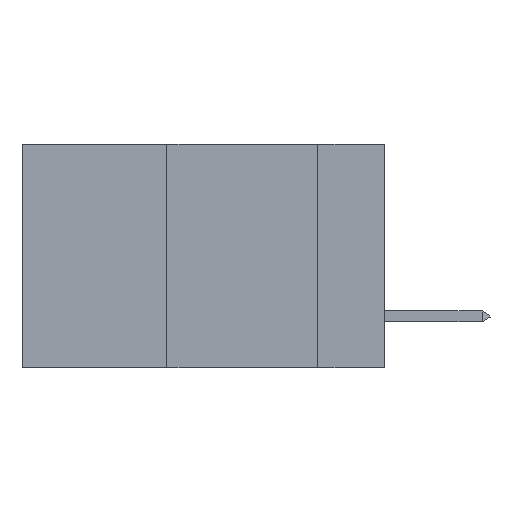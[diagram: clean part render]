
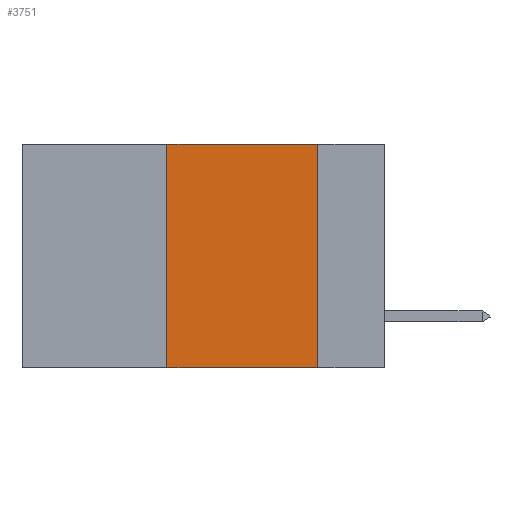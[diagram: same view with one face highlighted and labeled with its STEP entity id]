
A CAD part, left-side view. The second image highlights one B-rep face of the part: STEP entity #3751.
In plain terms, the highlighted planar face has unit normal (-1, 0, 0).
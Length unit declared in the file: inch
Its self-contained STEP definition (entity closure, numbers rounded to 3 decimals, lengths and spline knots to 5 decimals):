
#116 = DIRECTION ( 'NONE',  ( 0., 0., 1. ) ) ;
#193 = CARTESIAN_POINT ( 'NONE',  ( 0., 0.6, 0. ) ) ;
#438 = ORIENTED_EDGE ( 'NONE', *, *, #2894, .T. ) ;
#1217 = DIRECTION ( 'NONE',  ( 0., 0., -1. ) ) ;
#1274 = CARTESIAN_POINT ( 'NONE',  ( 0., 0.6, 0. ) ) ;
#1533 = DIRECTION ( 'NONE',  ( 0., -1., 0. ) ) ;
#1704 = EDGE_CURVE ( 'NONE', #3159, #12860, #2844, .T. ) ;
#2445 = LINE ( 'NONE', #13003, #3456 ) ;
#2676 = DIRECTION ( 'NONE',  ( 0., -1., 0. ) ) ;
#2844 = LINE ( 'NONE', #193, #10011 ) ;
#2891 = VERTEX_POINT ( 'NONE', #10988 ) ;
#2894 = EDGE_CURVE ( 'NONE', #2891, #12434, #9779, .T. ) ;
#3159 = VERTEX_POINT ( 'NONE', #9580 ) ;
#3456 = VECTOR ( 'NONE', #116, 39.37008 ) ;
#3751 = ADVANCED_FACE ( 'NONE', ( #7482 ), #6408, .F. ) ;
#3819 = DIRECTION ( 'NONE',  ( 0., 0., -1. ) ) ;
#6408 = PLANE ( 'NONE',  #15015 ) ;
#6765 = LINE ( 'NONE', #8893, #11883 ) ;
#7036 = ORIENTED_EDGE ( 'NONE', *, *, #13503, .F. ) ;
#7334 = ORIENTED_EDGE ( 'NONE', *, *, #1704, .F. ) ;
#7482 = FACE_OUTER_BOUND ( 'NONE', #8012, .T. ) ;
#7632 = CARTESIAN_POINT ( 'NONE',  ( 0., 0.11, -0.37 ) ) ;
#8012 = EDGE_LOOP ( 'NONE', ( #10747, #7334, #7036, #438 ) ) ;
#8443 = CARTESIAN_POINT ( 'NONE',  ( 0., 0.11, 0. ) ) ;
#8893 = CARTESIAN_POINT ( 'NONE',  ( 0., 0.11, 0. ) ) ;
#9580 = CARTESIAN_POINT ( 'NONE',  ( 0., 0.36, 0. ) ) ;
#9779 = LINE ( 'NONE', #12691, #16345 ) ;
#10011 = VECTOR ( 'NONE', #1533, 39.37008 ) ;
#10747 = ORIENTED_EDGE ( 'NONE', *, *, #12286, .F. ) ;
#10988 = CARTESIAN_POINT ( 'NONE',  ( 0., 0.36, -0.37 ) ) ;
#11883 = VECTOR ( 'NONE', #3819, 39.37008 ) ;
#12286 = EDGE_CURVE ( 'NONE', #12860, #12434, #6765, .T. ) ;
#12434 = VERTEX_POINT ( 'NONE', #7632 ) ;
#12691 = CARTESIAN_POINT ( 'NONE',  ( 0., 0.6, -0.37 ) ) ;
#12860 = VERTEX_POINT ( 'NONE', #8443 ) ;
#13003 = CARTESIAN_POINT ( 'NONE',  ( 0., 0.36, 0. ) ) ;
#13503 = EDGE_CURVE ( 'NONE', #2891, #3159, #2445, .T. ) ;
#15015 = AXIS2_PLACEMENT_3D ( 'NONE', #1274, #15590, #1217 ) ;
#15590 = DIRECTION ( 'NONE',  ( 1., 0., 0. ) ) ;
#16345 = VECTOR ( 'NONE', #2676, 39.37008 ) ;
